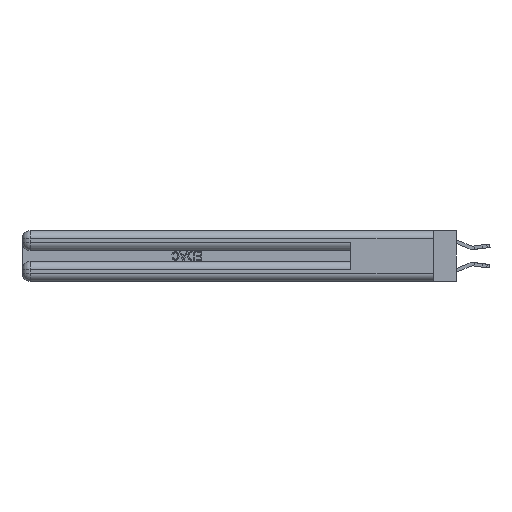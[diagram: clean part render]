
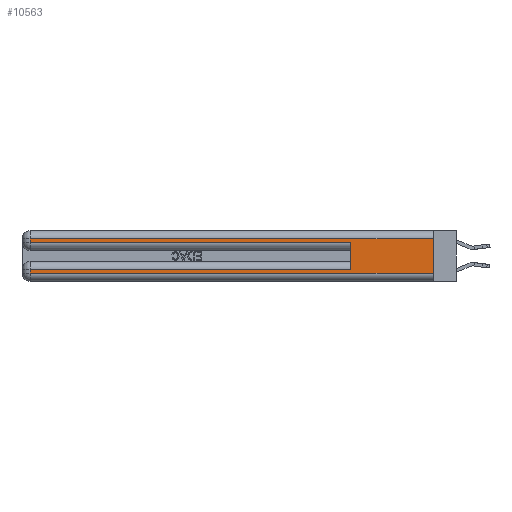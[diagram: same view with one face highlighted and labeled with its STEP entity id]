
A CAD part, left-side view. The second image highlights one B-rep face of the part: STEP entity #10563.
In plain terms, the highlighted planar face has unit normal (-1, 0, 0).
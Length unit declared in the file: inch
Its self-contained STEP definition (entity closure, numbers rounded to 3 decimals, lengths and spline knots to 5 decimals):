
#327 = EDGE_CURVE ( 'NONE', #731, #26238, #18651, .T. ) ;
#408 = DIRECTION ( 'NONE',  ( 0., 0., 1. ) ) ;
#731 = VERTEX_POINT ( 'NONE', #17760 ) ;
#1480 = CARTESIAN_POINT ( 'NONE',  ( 0., 0., 0.06 ) ) ;
#1700 = DIRECTION ( 'NONE',  ( 0., -1., 0. ) ) ;
#2064 = LINE ( 'NONE', #22449, #2759 ) ;
#2142 = VERTEX_POINT ( 'NONE', #20856 ) ;
#2758 = CARTESIAN_POINT ( 'NONE',  ( 0., 0., 0.31 ) ) ;
#2759 = VECTOR ( 'NONE', #7120, 39.37008 ) ;
#2794 = CARTESIAN_POINT ( 'NONE',  ( 0., 2.94, 0.37 ) ) ;
#2965 = LINE ( 'NONE', #1480, #8764 ) ;
#3243 = ORIENTED_EDGE ( 'NONE', *, *, #10963, .T. ) ;
#3642 = DIRECTION ( 'NONE',  ( 1., 0., 0. ) ) ;
#3654 = CARTESIAN_POINT ( 'NONE',  ( 0., 2.94, 0.285 ) ) ;
#3685 = EDGE_LOOP ( 'NONE', ( #25830, #3243, #20691, #15556, #27195, #16245, #5295, #18986 ) ) ;
#3703 = DIRECTION ( 'NONE',  ( 0., -1., 0. ) ) ;
#4695 = VECTOR ( 'NONE', #408, 39.37008 ) ;
#5295 = ORIENTED_EDGE ( 'NONE', *, *, #16021, .T. ) ;
#6712 = FACE_OUTER_BOUND ( 'NONE', #3685, .T. ) ;
#7120 = DIRECTION ( 'NONE',  ( 0., 0., -1. ) ) ;
#7699 = LINE ( 'NONE', #2794, #18666 ) ;
#8368 = VECTOR ( 'NONE', #25181, 39.37008 ) ;
#8547 = VERTEX_POINT ( 'NONE', #9541 ) ;
#8764 = VECTOR ( 'NONE', #3703, 39.37008 ) ;
#8832 = EDGE_CURVE ( 'NONE', #26238, #2142, #16682, .T. ) ;
#9541 = CARTESIAN_POINT ( 'NONE',  ( 0., 0., 0.06 ) ) ;
#9711 = VERTEX_POINT ( 'NONE', #28271 ) ;
#9845 = CARTESIAN_POINT ( 'NONE',  ( 0., 2.94, 0.37 ) ) ;
#10563 = ADVANCED_FACE ( 'NONE', ( #6712 ), #23238, .F. ) ;
#10851 = VECTOR ( 'NONE', #1700, 39.37008 ) ;
#10880 = EDGE_CURVE ( 'NONE', #12715, #2142, #27284, .T. ) ;
#10963 = EDGE_CURVE ( 'NONE', #15829, #731, #15652, .T. ) ;
#11253 = EDGE_CURVE ( 'NONE', #9711, #8547, #2965, .T. ) ;
#12715 = VERTEX_POINT ( 'NONE', #15349 ) ;
#13559 = CARTESIAN_POINT ( 'NONE',  ( 0., 0.6, 0.145 ) ) ;
#14528 = CARTESIAN_POINT ( 'NONE',  ( 0., 0., 0.37 ) ) ;
#14606 = LINE ( 'NONE', #26374, #25581 ) ;
#15349 = CARTESIAN_POINT ( 'NONE',  ( 0., 0.6, 0.085 ) ) ;
#15556 = ORIENTED_EDGE ( 'NONE', *, *, #8832, .T. ) ;
#15652 = LINE ( 'NONE', #2758, #20784 ) ;
#15829 = VERTEX_POINT ( 'NONE', #28353 ) ;
#16021 = EDGE_CURVE ( 'NONE', #26667, #9711, #7699, .T. ) ;
#16245 = ORIENTED_EDGE ( 'NONE', *, *, #25167, .T. ) ;
#16343 = CARTESIAN_POINT ( 'NONE',  ( 0., 2.94, 0.085 ) ) ;
#16682 = LINE ( 'NONE', #27816, #10851 ) ;
#17658 = DIRECTION ( 'NONE',  ( 0., 1., 0. ) ) ;
#17760 = CARTESIAN_POINT ( 'NONE',  ( 0., 2.94, 0.31 ) ) ;
#18651 = LINE ( 'NONE', #9845, #8368 ) ;
#18666 = VECTOR ( 'NONE', #20295, 39.37008 ) ;
#18933 = DIRECTION ( 'NONE',  ( 0., 0., -1. ) ) ;
#18986 = ORIENTED_EDGE ( 'NONE', *, *, #11253, .T. ) ;
#19805 = AXIS2_PLACEMENT_3D ( 'NONE', #14528, #3642, #18933 ) ;
#20260 = DIRECTION ( 'NONE',  ( 0., 1., 0. ) ) ;
#20295 = DIRECTION ( 'NONE',  ( 0., 0., -1. ) ) ;
#20691 = ORIENTED_EDGE ( 'NONE', *, *, #327, .T. ) ;
#20784 = VECTOR ( 'NONE', #20260, 39.37008 ) ;
#20856 = CARTESIAN_POINT ( 'NONE',  ( 0., 0.6, 0.285 ) ) ;
#22449 = CARTESIAN_POINT ( 'NONE',  ( 0., 0., 0.37 ) ) ;
#23070 = EDGE_CURVE ( 'NONE', #15829, #8547, #2064, .T. ) ;
#23238 = PLANE ( 'NONE',  #19805 ) ;
#25167 = EDGE_CURVE ( 'NONE', #12715, #26667, #14606, .T. ) ;
#25181 = DIRECTION ( 'NONE',  ( 0., 0., -1. ) ) ;
#25581 = VECTOR ( 'NONE', #17658, 39.37008 ) ;
#25830 = ORIENTED_EDGE ( 'NONE', *, *, #23070, .F. ) ;
#26238 = VERTEX_POINT ( 'NONE', #3654 ) ;
#26374 = CARTESIAN_POINT ( 'NONE',  ( 0., 0., 0.085 ) ) ;
#26667 = VERTEX_POINT ( 'NONE', #16343 ) ;
#27195 = ORIENTED_EDGE ( 'NONE', *, *, #10880, .F. ) ;
#27284 = LINE ( 'NONE', #13559, #4695 ) ;
#27816 = CARTESIAN_POINT ( 'NONE',  ( 0., 0., 0.285 ) ) ;
#28271 = CARTESIAN_POINT ( 'NONE',  ( 0., 2.94, 0.06 ) ) ;
#28353 = CARTESIAN_POINT ( 'NONE',  ( 0., 0., 0.31 ) ) ;
